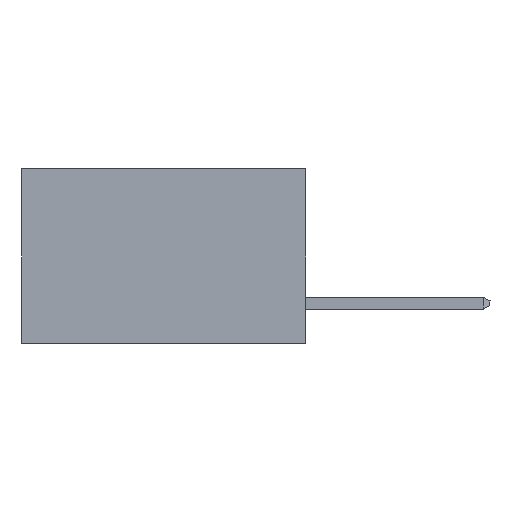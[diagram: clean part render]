
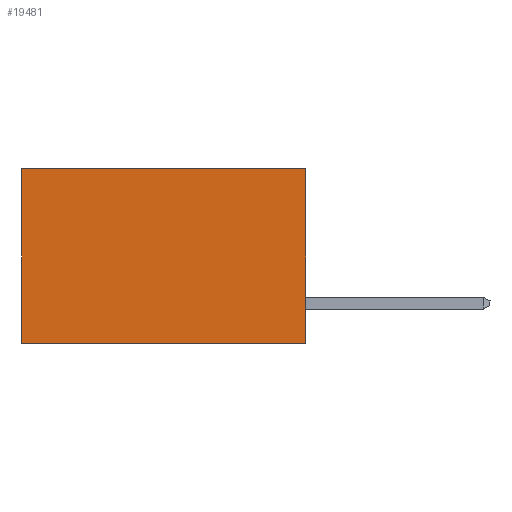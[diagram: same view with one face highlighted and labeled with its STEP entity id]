
A CAD part, left-side view. The second image highlights one B-rep face of the part: STEP entity #19481.
In plain terms, the highlighted planar face has unit normal (-1, 0, 0).
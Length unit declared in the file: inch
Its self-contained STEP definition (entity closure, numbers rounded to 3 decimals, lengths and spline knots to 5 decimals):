
#210 = VECTOR ( 'NONE', #15137, 39.37008 ) ;
#404 = ORIENTED_EDGE ( 'NONE', *, *, #3369, .F. ) ;
#1592 = VECTOR ( 'NONE', #9587, 39.37008 ) ;
#1817 = LINE ( 'NONE', #4501, #210 ) ;
#3087 = VERTEX_POINT ( 'NONE', #16987 ) ;
#3369 = EDGE_CURVE ( 'NONE', #11645, #17940, #13278, .T. ) ;
#3507 = LINE ( 'NONE', #18527, #1592 ) ;
#4052 = FACE_OUTER_BOUND ( 'NONE', #10438, .T. ) ;
#4501 = CARTESIAN_POINT ( 'NONE',  ( 0.2615, 0.6, -0.37 ) ) ;
#4845 = ORIENTED_EDGE ( 'NONE', *, *, #9474, .T. ) ;
#5019 = VECTOR ( 'NONE', #16168, 39.37008 ) ;
#6217 = EDGE_CURVE ( 'NONE', #11167, #3087, #11751, .T. ) ;
#6992 = VECTOR ( 'NONE', #8621, 39.37008 ) ;
#7356 = CARTESIAN_POINT ( 'NONE',  ( 0.2615, 0., -0.37 ) ) ;
#8516 = CARTESIAN_POINT ( 'NONE',  ( 0.2615, 0., 0. ) ) ;
#8621 = DIRECTION ( 'NONE',  ( 0., 1., 0. ) ) ;
#8842 = DIRECTION ( 'NONE',  ( 1., 0., 0. ) ) ;
#9474 = EDGE_CURVE ( 'NONE', #3087, #17940, #1817, .T. ) ;
#9587 = DIRECTION ( 'NONE',  ( 0., 0., -1. ) ) ;
#10056 = CARTESIAN_POINT ( 'NONE',  ( 0.2615, 0., -0.37 ) ) ;
#10438 = EDGE_LOOP ( 'NONE', ( #4845, #404, #18595, #17102 ) ) ;
#11167 = VERTEX_POINT ( 'NONE', #14647 ) ;
#11506 = DIRECTION ( 'NONE',  ( 0., 0., -1. ) ) ;
#11645 = VERTEX_POINT ( 'NONE', #7356 ) ;
#11751 = LINE ( 'NONE', #8516, #6992 ) ;
#12405 = CARTESIAN_POINT ( 'NONE',  ( 0.2615, 0.6, -0.37 ) ) ;
#13278 = LINE ( 'NONE', #19190, #5019 ) ;
#13975 = EDGE_CURVE ( 'NONE', #11167, #11645, #3507, .T. ) ;
#14647 = CARTESIAN_POINT ( 'NONE',  ( 0.2615, 0., 0. ) ) ;
#14718 = AXIS2_PLACEMENT_3D ( 'NONE', #10056, #8842, #11506 ) ;
#15137 = DIRECTION ( 'NONE',  ( 0., 0., -1. ) ) ;
#16168 = DIRECTION ( 'NONE',  ( 0., 1., 0. ) ) ;
#16987 = CARTESIAN_POINT ( 'NONE',  ( 0.2615, 0.6, 0. ) ) ;
#17102 = ORIENTED_EDGE ( 'NONE', *, *, #6217, .T. ) ;
#17590 = PLANE ( 'NONE',  #14718 ) ;
#17940 = VERTEX_POINT ( 'NONE', #12405 ) ;
#18527 = CARTESIAN_POINT ( 'NONE',  ( 0.2615, 0., -0.37 ) ) ;
#18595 = ORIENTED_EDGE ( 'NONE', *, *, #13975, .F. ) ;
#19190 = CARTESIAN_POINT ( 'NONE',  ( 0.2615, 0., -0.37 ) ) ;
#19481 = ADVANCED_FACE ( 'NONE', ( #4052 ), #17590, .F. ) ;
